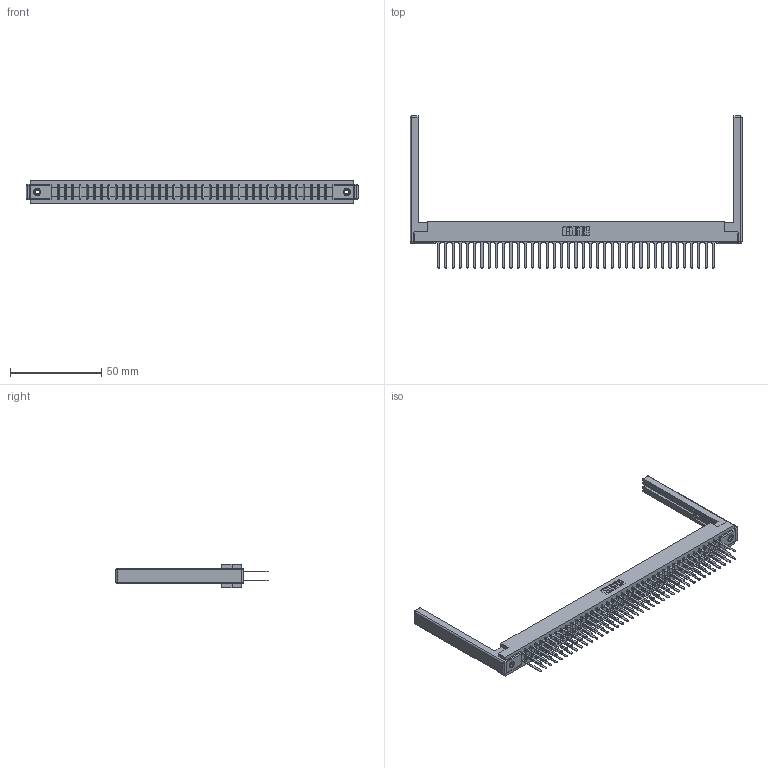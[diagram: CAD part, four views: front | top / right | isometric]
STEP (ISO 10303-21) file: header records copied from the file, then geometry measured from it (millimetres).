
FILE_DESCRIPTION (( 'STEP AP203' ), '1' );
FILE_NAME ('307-078-442-268.STEP', '2020-10-01T07:04:28', ( '' ), ( '' ), 'SwSTEP 2.0', 'SolidWorks 2020', '' );
FILE_SCHEMA (( 'CONFIG_CONTROL_DESIGN' ));
Length unit declared in the file: inch
Products named in the file (5): 307 Part_.156 Dia Mounting Holes; 307-078-442-268; 307-290-001_542; 307-220-068; 345-250-001_345-250-001-102
Assembly tree (83 placements, depth 2):
  307-078-442-268
    307 Part_.156 Dia Mounting Holes
    307-290-001_542  x78
    307-220-068  x2
    345-250-001_345-250-001-102  x2
Bounding box: 181.97 x 83.39 x 12.7 mm (x, y, z)
Volume: 24007.2 mm3; surface area: 29636.8 mm2
Topology: 83 solids, 83 shells, 3900 faces, 10853 edges, 7002 vertices
Faces by surface type: plane 2576, cylinder 1220, sphere 88, cone 12, torus 4
Entity records: 37779 total; most frequent: CARTESIAN_POINT 6156, ORIENTED_EDGE 6092, DIRECTION 6046, EDGE_CURVE 3046, LINE 2334, VECTOR 2334, VERTEX_POINT 1966, AXIS2_PLACEMENT_3D 1856
